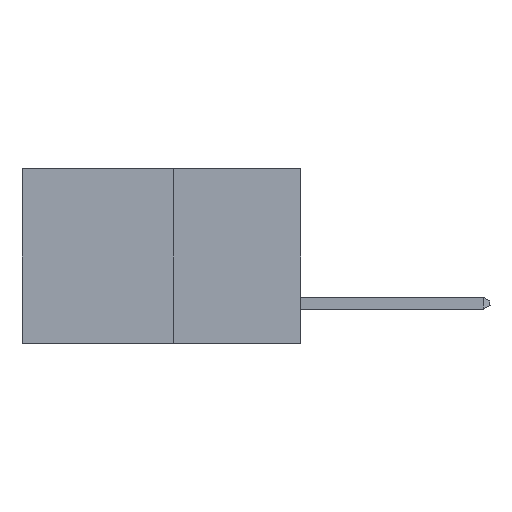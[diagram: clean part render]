
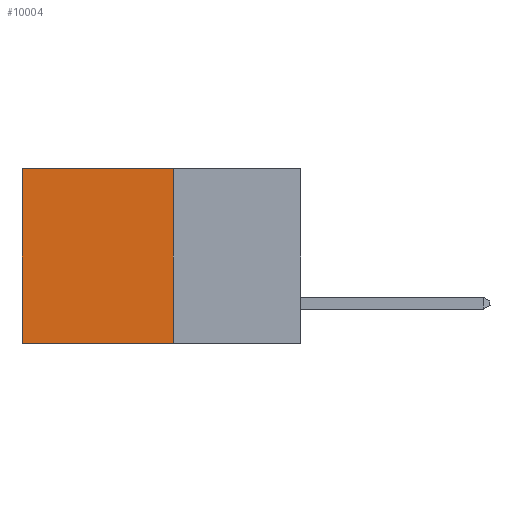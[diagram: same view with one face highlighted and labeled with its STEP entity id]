
A CAD part, left-side view. The second image highlights one B-rep face of the part: STEP entity #10004.
In plain terms, the highlighted planar face has unit normal (-1, 0, 0).
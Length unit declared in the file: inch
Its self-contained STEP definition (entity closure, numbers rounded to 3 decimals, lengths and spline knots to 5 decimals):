
#312 = VERTEX_POINT ( 'NONE', #6197 ) ;
#1726 = VECTOR ( 'NONE', #8737, 39.37008 ) ;
#2331 = VECTOR ( 'NONE', #11859, 39.37008 ) ;
#2398 = CARTESIAN_POINT ( 'NONE',  ( 0.277, 0.27, -0.37 ) ) ;
#2726 = LINE ( 'NONE', #2398, #2331 ) ;
#3036 = VERTEX_POINT ( 'NONE', #12451 ) ;
#3056 = VERTEX_POINT ( 'NONE', #9570 ) ;
#3326 = EDGE_CURVE ( 'NONE', #3036, #3056, #6974, .T. ) ;
#3378 = VECTOR ( 'NONE', #8808, 39.37008 ) ;
#3798 = VERTEX_POINT ( 'NONE', #13115 ) ;
#5133 = EDGE_CURVE ( 'NONE', #312, #3036, #7418, .T. ) ;
#5727 = PLANE ( 'NONE',  #12481 ) ;
#5763 = FACE_OUTER_BOUND ( 'NONE', #7055, .T. ) ;
#6197 = CARTESIAN_POINT ( 'NONE',  ( 0.277, 0.27, 0. ) ) ;
#6459 = ORIENTED_EDGE ( 'NONE', *, *, #13715, .F. ) ;
#6593 = LINE ( 'NONE', #8045, #3378 ) ;
#6956 = DIRECTION ( 'NONE',  ( 1., 0., 0. ) ) ;
#6974 = LINE ( 'NONE', #13199, #7748 ) ;
#7055 = EDGE_LOOP ( 'NONE', ( #7731, #6459, #9830, #12379 ) ) ;
#7418 = LINE ( 'NONE', #7552, #1726 ) ;
#7552 = CARTESIAN_POINT ( 'NONE',  ( 0.277, 0.27, 0. ) ) ;
#7731 = ORIENTED_EDGE ( 'NONE', *, *, #3326, .T. ) ;
#7748 = VECTOR ( 'NONE', #13273, 39.37008 ) ;
#8045 = CARTESIAN_POINT ( 'NONE',  ( 0.277, 0.27, -0.37 ) ) ;
#8737 = DIRECTION ( 'NONE',  ( 0., 1., 0. ) ) ;
#8808 = DIRECTION ( 'NONE',  ( 0., 1., 0. ) ) ;
#9550 = EDGE_CURVE ( 'NONE', #312, #3798, #2726, .T. ) ;
#9570 = CARTESIAN_POINT ( 'NONE',  ( 0.277, 0.59, -0.37 ) ) ;
#9830 = ORIENTED_EDGE ( 'NONE', *, *, #9550, .F. ) ;
#10004 = ADVANCED_FACE ( 'NONE', ( #5763 ), #5727, .F. ) ;
#11859 = DIRECTION ( 'NONE',  ( 0., 0., -1. ) ) ;
#12379 = ORIENTED_EDGE ( 'NONE', *, *, #5133, .T. ) ;
#12451 = CARTESIAN_POINT ( 'NONE',  ( 0.277, 0.59, 0. ) ) ;
#12481 = AXIS2_PLACEMENT_3D ( 'NONE', #13783, #6956, #14884 ) ;
#13115 = CARTESIAN_POINT ( 'NONE',  ( 0.277, 0.27, -0.37 ) ) ;
#13199 = CARTESIAN_POINT ( 'NONE',  ( 0.277, 0.59, -0.37 ) ) ;
#13273 = DIRECTION ( 'NONE',  ( 0., 0., -1. ) ) ;
#13715 = EDGE_CURVE ( 'NONE', #3798, #3056, #6593, .T. ) ;
#13783 = CARTESIAN_POINT ( 'NONE',  ( 0.277, 0.27, -0.37 ) ) ;
#14884 = DIRECTION ( 'NONE',  ( 0., 0., -1. ) ) ;
